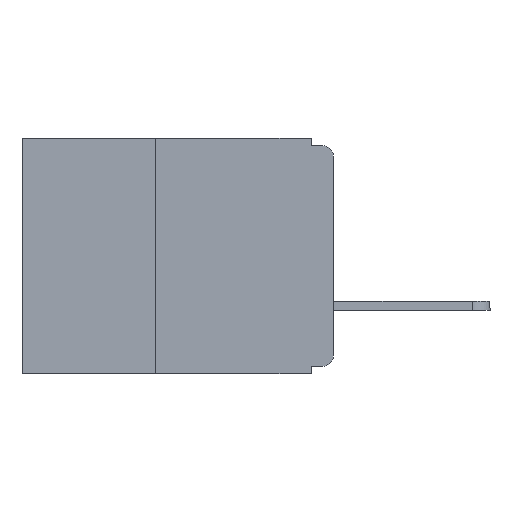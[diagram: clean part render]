
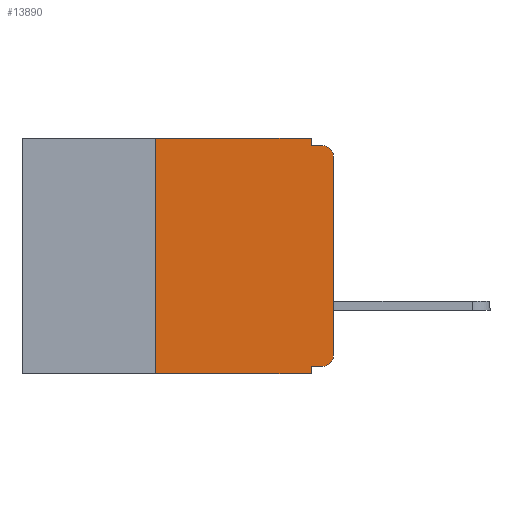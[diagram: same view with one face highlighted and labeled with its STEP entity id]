
A CAD part, left-side view. The second image highlights one B-rep face of the part: STEP entity #13890.
In plain terms, the highlighted planar face has unit normal (-1, 0, 0).
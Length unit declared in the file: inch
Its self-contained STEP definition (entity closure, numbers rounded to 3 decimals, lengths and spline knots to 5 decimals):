
#429 = ORIENTED_EDGE ( 'NONE', *, *, #13034, .T. ) ;
#538 = DIRECTION ( 'NONE',  ( 0., -1., 0. ) ) ;
#541 = ORIENTED_EDGE ( 'NONE', *, *, #3991, .T. ) ;
#654 = DIRECTION ( 'NONE',  ( 0., -1., 0. ) ) ;
#719 = CARTESIAN_POINT ( 'NONE',  ( 0., 0., -0.01 ) ) ;
#1308 = LINE ( 'NONE', #5054, #1322 ) ;
#1322 = VECTOR ( 'NONE', #5322, 39.37008 ) ;
#1493 = CARTESIAN_POINT ( 'NONE',  ( 0., 0.437, -0.33 ) ) ;
#2367 = ORIENTED_EDGE ( 'NONE', *, *, #11800, .T. ) ;
#2575 = ORIENTED_EDGE ( 'NONE', *, *, #18940, .F. ) ;
#2619 = DIRECTION ( 'NONE',  ( 0., 0., -1. ) ) ;
#2639 = EDGE_LOOP ( 'NONE', ( #2367, #541, #9123, #16688, #2575, #3382, #11111, #11604, #2993, #429 ) ) ;
#2825 = CARTESIAN_POINT ( 'NONE',  ( 0., 0.437, 0. ) ) ;
#2993 = ORIENTED_EDGE ( 'NONE', *, *, #17495, .F. ) ;
#3055 = LINE ( 'NONE', #719, #3332 ) ;
#3332 = VECTOR ( 'NONE', #654, 39.37008 ) ;
#3382 = ORIENTED_EDGE ( 'NONE', *, *, #15677, .F. ) ;
#3400 = CARTESIAN_POINT ( 'NONE',  ( 0., 0.25, -0.33 ) ) ;
#3609 = DIRECTION ( 'NONE',  ( 0., 0., 1. ) ) ;
#3689 = AXIS2_PLACEMENT_3D ( 'NONE', #2825, #10253, #2619 ) ;
#3991 = EDGE_CURVE ( 'NONE', #13024, #8538, #4093, .T. ) ;
#4093 = CIRCLE ( 'NONE', #14077, 0.015 ) ;
#4256 = CARTESIAN_POINT ( 'NONE',  ( 0., 0., -0.305 ) ) ;
#4522 = VERTEX_POINT ( 'NONE', #6949 ) ;
#5054 = CARTESIAN_POINT ( 'NONE',  ( 0., 0.437, 0. ) ) ;
#5204 = EDGE_CURVE ( 'NONE', #12447, #11823, #12727, .T. ) ;
#5322 = DIRECTION ( 'NONE',  ( 0., -1., 0. ) ) ;
#5533 = DIRECTION ( 'NONE',  ( 0., 1., 0. ) ) ;
#6062 = VECTOR ( 'NONE', #3609, 39.37008 ) ;
#6085 = LINE ( 'NONE', #3400, #6062 ) ;
#6266 = CARTESIAN_POINT ( 'NONE',  ( 0., 0.015, -0.01 ) ) ;
#6271 = CARTESIAN_POINT ( 'NONE',  ( 0., 0., -0.32 ) ) ;
#6872 = EDGE_CURVE ( 'NONE', #14174, #8538, #3055, .T. ) ;
#6949 = CARTESIAN_POINT ( 'NONE',  ( 0., 0.015, -0.32 ) ) ;
#7081 = CARTESIAN_POINT ( 'NONE',  ( 0., 0.25, 0. ) ) ;
#7273 = LINE ( 'NONE', #14483, #7666 ) ;
#7666 = VECTOR ( 'NONE', #13217, 39.37008 ) ;
#7719 = EDGE_CURVE ( 'NONE', #17065, #14174, #17680, .T. ) ;
#7880 = VERTEX_POINT ( 'NONE', #4256 ) ;
#8295 = DIRECTION ( 'NONE',  ( 0., 0., -1. ) ) ;
#8538 = VERTEX_POINT ( 'NONE', #6266 ) ;
#8541 = CARTESIAN_POINT ( 'NONE',  ( 0., 0.031, -0.01 ) ) ;
#9123 = ORIENTED_EDGE ( 'NONE', *, *, #6872, .F. ) ;
#9129 = CARTESIAN_POINT ( 'NONE',  ( 0., 0.25, -0.33 ) ) ;
#9182 = CARTESIAN_POINT ( 'NONE',  ( 0., 0.031, 0. ) ) ;
#9323 = CARTESIAN_POINT ( 'NONE',  ( 0., 0.015, -0.025 ) ) ;
#9753 = AXIS2_PLACEMENT_3D ( 'NONE', #15069, #15132, #14526 ) ;
#10253 = DIRECTION ( 'NONE',  ( 1., 0., 0. ) ) ;
#11111 = ORIENTED_EDGE ( 'NONE', *, *, #5204, .T. ) ;
#11410 = DIRECTION ( 'NONE',  ( -1., 0., 0. ) ) ;
#11604 = ORIENTED_EDGE ( 'NONE', *, *, #16995, .F. ) ;
#11724 = DIRECTION ( 'NONE',  ( 0., 0., -1. ) ) ;
#11800 = EDGE_CURVE ( 'NONE', #7880, #13024, #7273, .T. ) ;
#11823 = VERTEX_POINT ( 'NONE', #12841 ) ;
#11889 = CARTESIAN_POINT ( 'NONE',  ( 0., 0.031, -0.33 ) ) ;
#12313 = VECTOR ( 'NONE', #5533, 39.37008 ) ;
#12431 = LINE ( 'NONE', #6271, #12313 ) ;
#12447 = VERTEX_POINT ( 'NONE', #9129 ) ;
#12639 = VECTOR ( 'NONE', #538, 39.37008 ) ;
#12727 = LINE ( 'NONE', #1493, #12639 ) ;
#12841 = CARTESIAN_POINT ( 'NONE',  ( 0., 0.031, -0.33 ) ) ;
#12941 = VERTEX_POINT ( 'NONE', #7081 ) ;
#13024 = VERTEX_POINT ( 'NONE', #16125 ) ;
#13034 = EDGE_CURVE ( 'NONE', #4522, #7880, #14859, .T. ) ;
#13217 = DIRECTION ( 'NONE',  ( 0., 0., 1. ) ) ;
#13890 = ADVANCED_FACE ( 'NONE', ( #14095 ), #18393, .F. ) ;
#14077 = AXIS2_PLACEMENT_3D ( 'NONE', #9323, #11410, #8295 ) ;
#14095 = FACE_OUTER_BOUND ( 'NONE', #2639, .T. ) ;
#14167 = CARTESIAN_POINT ( 'NONE',  ( 0., 0.031, 0. ) ) ;
#14174 = VERTEX_POINT ( 'NONE', #8541 ) ;
#14207 = DIRECTION ( 'NONE',  ( 0., 0., -1. ) ) ;
#14483 = CARTESIAN_POINT ( 'NONE',  ( 0., 0., 0. ) ) ;
#14526 = DIRECTION ( 'NONE',  ( 0., 0., -1. ) ) ;
#14859 = CIRCLE ( 'NONE', #9753, 0.015 ) ;
#15069 = CARTESIAN_POINT ( 'NONE',  ( 0., 0.015, -0.305 ) ) ;
#15132 = DIRECTION ( 'NONE',  ( -1., 0., 0. ) ) ;
#15677 = EDGE_CURVE ( 'NONE', #12447, #12941, #6085, .T. ) ;
#16125 = CARTESIAN_POINT ( 'NONE',  ( 0., 0., -0.025 ) ) ;
#16553 = CARTESIAN_POINT ( 'NONE',  ( 0., 0.031, -0.32 ) ) ;
#16578 = VECTOR ( 'NONE', #11724, 39.37008 ) ;
#16688 = ORIENTED_EDGE ( 'NONE', *, *, #7719, .F. ) ;
#16776 = LINE ( 'NONE', #11889, #16578 ) ;
#16995 = EDGE_CURVE ( 'NONE', #19064, #11823, #16776, .T. ) ;
#17065 = VERTEX_POINT ( 'NONE', #9182 ) ;
#17495 = EDGE_CURVE ( 'NONE', #4522, #19064, #12431, .T. ) ;
#17680 = LINE ( 'NONE', #14167, #17769 ) ;
#17769 = VECTOR ( 'NONE', #14207, 39.37008 ) ;
#18393 = PLANE ( 'NONE',  #3689 ) ;
#18940 = EDGE_CURVE ( 'NONE', #12941, #17065, #1308, .T. ) ;
#19064 = VERTEX_POINT ( 'NONE', #16553 ) ;
